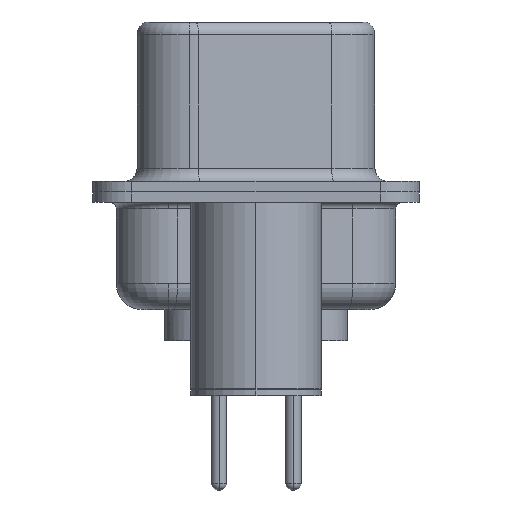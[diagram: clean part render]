
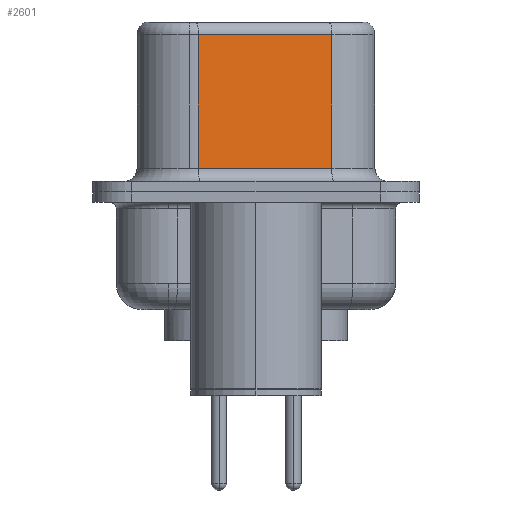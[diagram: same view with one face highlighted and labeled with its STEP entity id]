
A CAD part, left-side view. The second image highlights one B-rep face of the part: STEP entity #2601.
In plain terms, the highlighted planar face has unit normal (-0.985, -0.174, 0).
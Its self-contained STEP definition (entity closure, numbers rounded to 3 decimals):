
#519 = EDGE_LOOP ( 'NONE', ( #17811, #7890, #7328, #16865 ) ) ;
#832 = LINE ( 'NONE', #5906, #8186 ) ;
#1255 = VECTOR ( 'NONE', #10557, 1000. ) ;
#1360 = CARTESIAN_POINT ( 'NONE',  ( 4.58, -2.897, 6.02 ) ) ;
#1598 = FACE_OUTER_BOUND ( 'NONE', #519, .T. ) ;
#2341 = CARTESIAN_POINT ( 'NONE',  ( 4.58, -2.897, 0.9 ) ) ;
#2601 = ADVANCED_FACE ( 'NONE', ( #1598 ), #2917, .F. ) ;
#2917 = PLANE ( 'NONE',  #4494 ) ;
#3757 = LINE ( 'NONE', #2341, #11396 ) ;
#4494 = AXIS2_PLACEMENT_3D ( 'NONE', #6372, #11087, #21059 ) ;
#5611 = CARTESIAN_POINT ( 'NONE',  ( 3.68, 2.203, 6.52 ) ) ;
#5906 = CARTESIAN_POINT ( 'NONE',  ( 4.58, -2.897, 6.52 ) ) ;
#6372 = CARTESIAN_POINT ( 'NONE',  ( 4.58, -2.897, 6.52 ) ) ;
#6986 = EDGE_CURVE ( 'NONE', #8693, #19703, #832, .T. ) ;
#7133 = EDGE_CURVE ( 'NONE', #8693, #7616, #13017, .T. ) ;
#7328 = ORIENTED_EDGE ( 'NONE', *, *, #17340, .T. ) ;
#7616 = VERTEX_POINT ( 'NONE', #12883 ) ;
#7890 = ORIENTED_EDGE ( 'NONE', *, *, #7133, .T. ) ;
#8186 = VECTOR ( 'NONE', #10629, 1000. ) ;
#8548 = CARTESIAN_POINT ( 'NONE',  ( 3.68, 2.203, 0.9 ) ) ;
#8693 = VERTEX_POINT ( 'NONE', #1360 ) ;
#10557 = DIRECTION ( 'NONE',  ( 0., 0., -1. ) ) ;
#10629 = DIRECTION ( 'NONE',  ( 0., 0., -1. ) ) ;
#11087 = DIRECTION ( 'NONE',  ( 0.985, 0.174, 0. ) ) ;
#11267 = CARTESIAN_POINT ( 'NONE',  ( 4.58, -2.897, 6.02 ) ) ;
#11396 = VECTOR ( 'NONE', #15603, 1000. ) ;
#11967 = LINE ( 'NONE', #5611, #1255 ) ;
#12654 = EDGE_CURVE ( 'NONE', #15612, #19703, #3757, .T. ) ;
#12883 = CARTESIAN_POINT ( 'NONE',  ( 3.68, 2.203, 6.02 ) ) ;
#13017 = LINE ( 'NONE', #11267, #14055 ) ;
#14055 = VECTOR ( 'NONE', #17756, 1000. ) ;
#15603 = DIRECTION ( 'NONE',  ( 0.174, -0.985, 0. ) ) ;
#15612 = VERTEX_POINT ( 'NONE', #8548 ) ;
#16865 = ORIENTED_EDGE ( 'NONE', *, *, #12654, .T. ) ;
#17340 = EDGE_CURVE ( 'NONE', #7616, #15612, #11967, .T. ) ;
#17756 = DIRECTION ( 'NONE',  ( -0.174, 0.985, 0. ) ) ;
#17811 = ORIENTED_EDGE ( 'NONE', *, *, #6986, .F. ) ;
#19703 = VERTEX_POINT ( 'NONE', #20887 ) ;
#20887 = CARTESIAN_POINT ( 'NONE',  ( 4.58, -2.897, 0.9 ) ) ;
#21059 = DIRECTION ( 'NONE',  ( -0.174, 0.985, 0. ) ) ;
